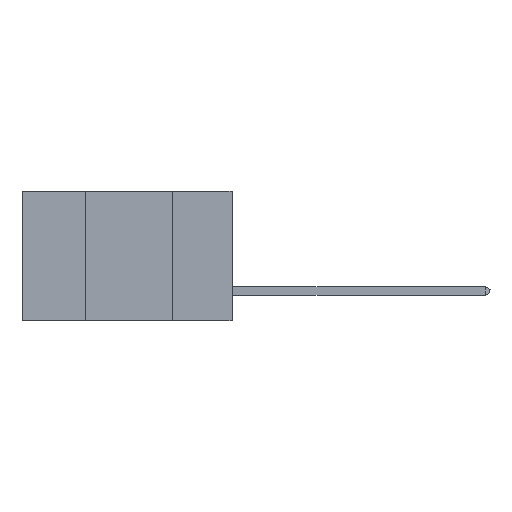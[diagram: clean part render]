
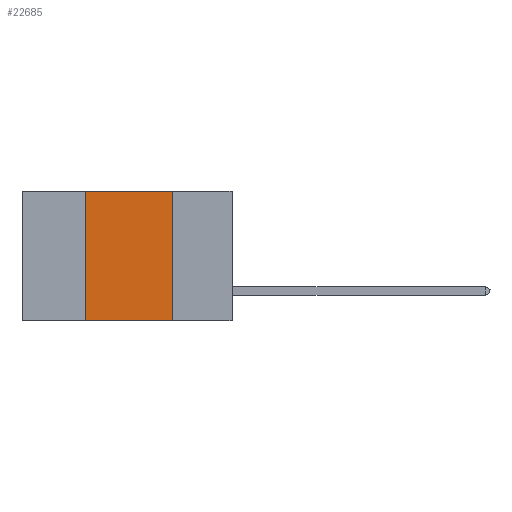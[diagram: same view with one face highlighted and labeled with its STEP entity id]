
A CAD part, left-side view. The second image highlights one B-rep face of the part: STEP entity #22685.
In plain terms, the highlighted planar face has unit normal (-1, 0, 0).
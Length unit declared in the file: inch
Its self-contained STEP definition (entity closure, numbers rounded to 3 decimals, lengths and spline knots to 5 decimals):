
#463 = CARTESIAN_POINT ( 'NONE',  ( 0., 0.17, 0. ) ) ;
#4420 = VECTOR ( 'NONE', #9579, 39.37008 ) ;
#5039 = DIRECTION ( 'NONE',  ( 0., 0., 1. ) ) ;
#5203 = VECTOR ( 'NONE', #10985, 39.37008 ) ;
#5839 = CARTESIAN_POINT ( 'NONE',  ( 0., 0.42, 0. ) ) ;
#6089 = VERTEX_POINT ( 'NONE', #28579 ) ;
#6152 = DIRECTION ( 'NONE',  ( 0., 0., -1. ) ) ;
#6189 = CARTESIAN_POINT ( 'NONE',  ( 0., 0.42, -0.37 ) ) ;
#8690 = AXIS2_PLACEMENT_3D ( 'NONE', #41167, #27956, #6152 ) ;
#9464 = VERTEX_POINT ( 'NONE', #463 ) ;
#9579 = DIRECTION ( 'NONE',  ( 0., 0., -1. ) ) ;
#10054 = VECTOR ( 'NONE', #40898, 39.37008 ) ;
#10985 = DIRECTION ( 'NONE',  ( 0., -1., 0. ) ) ;
#13925 = LINE ( 'NONE', #26723, #5203 ) ;
#14764 = VERTEX_POINT ( 'NONE', #6189 ) ;
#15079 = LINE ( 'NONE', #34580, #18117 ) ;
#15584 = FACE_OUTER_BOUND ( 'NONE', #23566, .T. ) ;
#17842 = LINE ( 'NONE', #24551, #10054 ) ;
#18117 = VECTOR ( 'NONE', #5039, 39.37008 ) ;
#18812 = LINE ( 'NONE', #28256, #4420 ) ;
#20965 = EDGE_CURVE ( 'NONE', #24735, #9464, #17842, .T. ) ;
#22304 = PLANE ( 'NONE',  #8690 ) ;
#22685 = ADVANCED_FACE ( 'NONE', ( #15584 ), #22304, .F. ) ;
#22770 = ORIENTED_EDGE ( 'NONE', *, *, #20965, .F. ) ;
#23566 = EDGE_LOOP ( 'NONE', ( #37039, #22770, #28642, #24651 ) ) ;
#24551 = CARTESIAN_POINT ( 'NONE',  ( 0., 0.6, 0. ) ) ;
#24651 = ORIENTED_EDGE ( 'NONE', *, *, #37550, .T. ) ;
#24735 = VERTEX_POINT ( 'NONE', #5839 ) ;
#26723 = CARTESIAN_POINT ( 'NONE',  ( 0., 0.6, -0.37 ) ) ;
#27956 = DIRECTION ( 'NONE',  ( 1., 0., 0. ) ) ;
#28256 = CARTESIAN_POINT ( 'NONE',  ( 0., 0.17, 0. ) ) ;
#28579 = CARTESIAN_POINT ( 'NONE',  ( 0., 0.17, -0.37 ) ) ;
#28598 = EDGE_CURVE ( 'NONE', #9464, #6089, #18812, .T. ) ;
#28642 = ORIENTED_EDGE ( 'NONE', *, *, #35338, .F. ) ;
#34580 = CARTESIAN_POINT ( 'NONE',  ( 0., 0.42, 0. ) ) ;
#35338 = EDGE_CURVE ( 'NONE', #14764, #24735, #15079, .T. ) ;
#37039 = ORIENTED_EDGE ( 'NONE', *, *, #28598, .F. ) ;
#37550 = EDGE_CURVE ( 'NONE', #14764, #6089, #13925, .T. ) ;
#40898 = DIRECTION ( 'NONE',  ( 0., -1., 0. ) ) ;
#41167 = CARTESIAN_POINT ( 'NONE',  ( 0., 0.6, 0. ) ) ;
